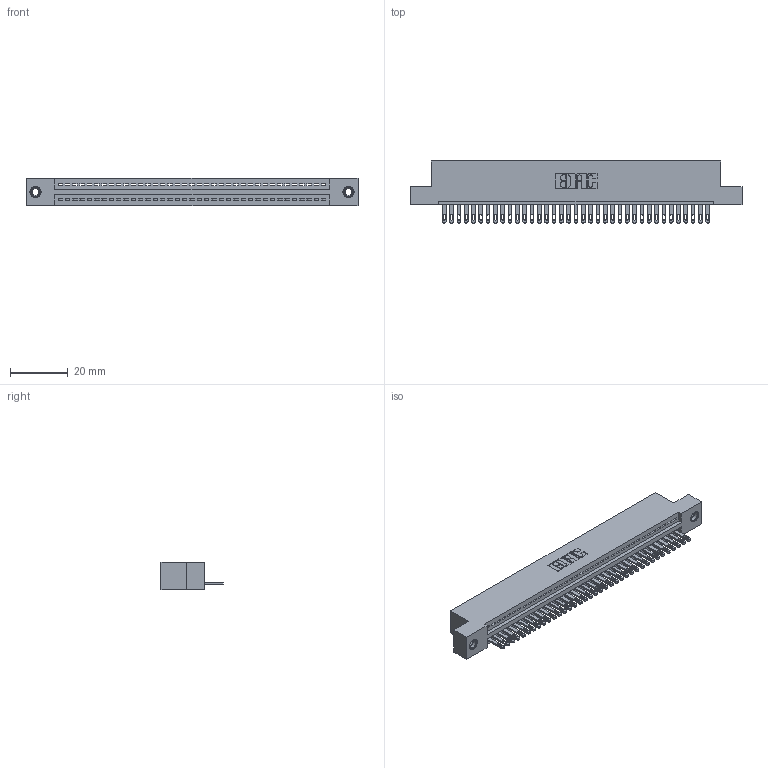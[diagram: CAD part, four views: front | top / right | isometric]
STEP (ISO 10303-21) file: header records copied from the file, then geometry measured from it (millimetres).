
FILE_DESCRIPTION (( 'STEP AP203' ), '1' );
FILE_NAME ('895-037-500-108.STEP', '2020-09-26T00:08:59', ( '' ), ( '' ), 'SwSTEP 2.0', 'SolidWorks 2020', '' );
FILE_SCHEMA (( 'CONFIG_CONTROL_DESIGN' ));
Length unit declared in the file: inch
Products named in the file (4): 845 Part_Flush Mounting Lugs - 0.156 Dia-TI; 895-037-500-108; 345-250-001_345-250-003-102; 345-292-001_345-293-100
Assembly tree (40 placements, depth 2):
  895-037-500-108
    845 Part_Flush Mounting Lugs - 0.156 Dia-TI
    345-292-001_345-293-100  x37
    345-250-001_345-250-003-102  x2
Bounding box: 115.19 x 21.51 x 9.4 mm (x, y, z)
Volume: 10916.2 mm3; surface area: 14540.9 mm2
Topology: 40 solids, 40 shells, 2184 faces, 6693 edges, 4454 vertices
Faces by surface type: plane 1370, cylinder 798, cone 12, torus 4
Entity records: 29636 total; most frequent: CARTESIAN_POINT 5114, ORIENTED_EDGE 5078, DIRECTION 4503, EDGE_CURVE 2539, VECTOR 2235, LINE 2235, VERTEX_POINT 1688, AXIS2_PLACEMENT_3D 1134
